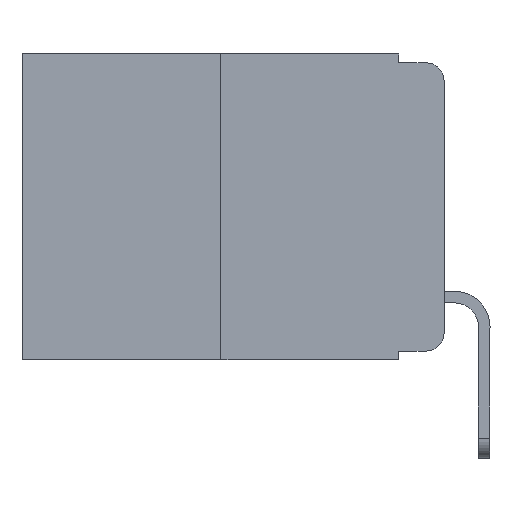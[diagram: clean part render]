
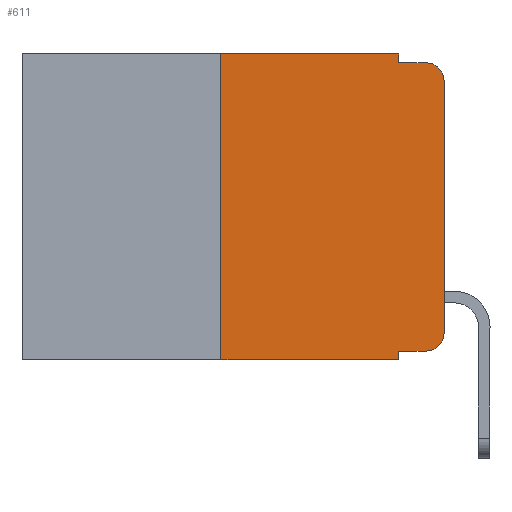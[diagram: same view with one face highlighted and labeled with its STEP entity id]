
A CAD part, left-side view. The second image highlights one B-rep face of the part: STEP entity #611.
In plain terms, the highlighted planar face has unit normal (-1, 0, 0).
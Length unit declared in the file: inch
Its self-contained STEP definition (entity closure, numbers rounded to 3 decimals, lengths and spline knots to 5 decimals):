
#88 = VECTOR ( 'NONE', #9686, 39.37008 ) ;
#611 = ADVANCED_FACE ( 'NONE', ( #10473 ), #3300, .F. ) ;
#733 = LINE ( 'NONE', #9210, #88 ) ;
#1097 = DIRECTION ( 'NONE',  ( 0., 0., 1. ) ) ;
#1259 = DIRECTION ( 'NONE',  ( -1., 0., 0. ) ) ;
#1465 = CARTESIAN_POINT ( 'NONE',  ( 0., 0.473, -0.343 ) ) ;
#1466 = EDGE_CURVE ( 'NONE', #6577, #6787, #733, .T. ) ;
#1718 = ORIENTED_EDGE ( 'NONE', *, *, #11756, .T. ) ;
#3211 = CARTESIAN_POINT ( 'NONE',  ( 0., 0.473, 0. ) ) ;
#3230 = VERTEX_POINT ( 'NONE', #4452 ) ;
#3300 = PLANE ( 'NONE',  #22395 ) ;
#3585 = ORIENTED_EDGE ( 'NONE', *, *, #6081, .T. ) ;
#3670 = LINE ( 'NONE', #19578, #22132 ) ;
#4152 = CARTESIAN_POINT ( 'NONE',  ( 0., 0.051, 0. ) ) ;
#4452 = CARTESIAN_POINT ( 'NONE',  ( 0., 0.051, -0.01 ) ) ;
#5296 = VERTEX_POINT ( 'NONE', #10024 ) ;
#5356 = CARTESIAN_POINT ( 'NONE',  ( 0., 0.02, -0.333 ) ) ;
#5412 = EDGE_CURVE ( 'NONE', #6280, #3230, #3670, .T. ) ;
#6081 = EDGE_CURVE ( 'NONE', #6577, #10014, #23718, .T. ) ;
#6172 = LINE ( 'NONE', #19785, #20274 ) ;
#6280 = VERTEX_POINT ( 'NONE', #22541 ) ;
#6577 = VERTEX_POINT ( 'NONE', #19228 ) ;
#6715 = EDGE_CURVE ( 'NONE', #3230, #21438, #17166, .T. ) ;
#6787 = VERTEX_POINT ( 'NONE', #16403 ) ;
#6849 = CARTESIAN_POINT ( 'NONE',  ( 0., 0.051, -0.01 ) ) ;
#6919 = ORIENTED_EDGE ( 'NONE', *, *, #9229, .T. ) ;
#6920 = DIRECTION ( 'NONE',  ( -1., 0., 0. ) ) ;
#7929 = LINE ( 'NONE', #4152, #16643 ) ;
#8415 = VECTOR ( 'NONE', #13838, 39.37008 ) ;
#9210 = CARTESIAN_POINT ( 'NONE',  ( 0., 0.25, 0. ) ) ;
#9229 = EDGE_CURVE ( 'NONE', #5296, #21438, #17628, .T. ) ;
#9271 = ORIENTED_EDGE ( 'NONE', *, *, #23041, .F. ) ;
#9686 = DIRECTION ( 'NONE',  ( 0., 0., 1. ) ) ;
#9834 = CARTESIAN_POINT ( 'NONE',  ( 0., 0.02, -0.01 ) ) ;
#9861 = ORIENTED_EDGE ( 'NONE', *, *, #18319, .T. ) ;
#10014 = VERTEX_POINT ( 'NONE', #17397 ) ;
#10024 = CARTESIAN_POINT ( 'NONE',  ( 0., 0., -0.03 ) ) ;
#10473 = FACE_OUTER_BOUND ( 'NONE', #21696, .T. ) ;
#11504 = DIRECTION ( 'NONE',  ( 0., -1., 0. ) ) ;
#11756 = EDGE_CURVE ( 'NONE', #23983, #5296, #6172, .T. ) ;
#11792 = DIRECTION ( 'NONE',  ( 0., 0., -1. ) ) ;
#11904 = ORIENTED_EDGE ( 'NONE', *, *, #6715, .F. ) ;
#12488 = ORIENTED_EDGE ( 'NONE', *, *, #5412, .F. ) ;
#12557 = CARTESIAN_POINT ( 'NONE',  ( 0., 0., -0.313 ) ) ;
#12733 = CARTESIAN_POINT ( 'NONE',  ( 0., 0.02, -0.03 ) ) ;
#13445 = CIRCLE ( 'NONE', #21872, 0.02 ) ;
#13838 = DIRECTION ( 'NONE',  ( 0., -1., 0. ) ) ;
#14300 = VECTOR ( 'NONE', #23679, 39.37008 ) ;
#14572 = LINE ( 'NONE', #15698, #8415 ) ;
#14627 = DIRECTION ( 'NONE',  ( 0., 0., -1. ) ) ;
#14845 = ORIENTED_EDGE ( 'NONE', *, *, #15960, .T. ) ;
#15241 = DIRECTION ( 'NONE',  ( 0., 0., -1. ) ) ;
#15698 = CARTESIAN_POINT ( 'NONE',  ( 0., 0.473, 0. ) ) ;
#15960 = EDGE_CURVE ( 'NONE', #22687, #23983, #13445, .T. ) ;
#16187 = DIRECTION ( 'NONE',  ( 1., 0., 0. ) ) ;
#16403 = CARTESIAN_POINT ( 'NONE',  ( 0., 0.25, 0. ) ) ;
#16643 = VECTOR ( 'NONE', #11792, 39.37008 ) ;
#16652 = VERTEX_POINT ( 'NONE', #23336 ) ;
#17031 = EDGE_CURVE ( 'NONE', #6787, #6280, #14572, .T. ) ;
#17166 = LINE ( 'NONE', #6849, #22403 ) ;
#17361 = ORIENTED_EDGE ( 'NONE', *, *, #17031, .F. ) ;
#17397 = CARTESIAN_POINT ( 'NONE',  ( 0., 0.051, -0.343 ) ) ;
#17628 = CIRCLE ( 'NONE', #20073, 0.02 ) ;
#17997 = CARTESIAN_POINT ( 'NONE',  ( 0., 0.02, -0.313 ) ) ;
#18319 = EDGE_CURVE ( 'NONE', #16652, #22687, #23109, .T. ) ;
#19228 = CARTESIAN_POINT ( 'NONE',  ( 0., 0.25, -0.343 ) ) ;
#19578 = CARTESIAN_POINT ( 'NONE',  ( 0., 0.051, 0. ) ) ;
#19717 = DIRECTION ( 'NONE',  ( 0., -1., 0. ) ) ;
#19773 = DIRECTION ( 'NONE',  ( 0., 0., -1. ) ) ;
#19785 = CARTESIAN_POINT ( 'NONE',  ( 0., 0., 0. ) ) ;
#20073 = AXIS2_PLACEMENT_3D ( 'NONE', #12733, #1259, #14627 ) ;
#20274 = VECTOR ( 'NONE', #1097, 39.37008 ) ;
#21384 = DIRECTION ( 'NONE',  ( 0., 0., -1. ) ) ;
#21438 = VERTEX_POINT ( 'NONE', #9834 ) ;
#21696 = EDGE_LOOP ( 'NONE', ( #1718, #6919, #11904, #12488, #17361, #22600, #3585, #9271, #9861, #14845 ) ) ;
#21872 = AXIS2_PLACEMENT_3D ( 'NONE', #17997, #6920, #19773 ) ;
#22020 = VECTOR ( 'NONE', #11504, 39.37008 ) ;
#22132 = VECTOR ( 'NONE', #21384, 39.37008 ) ;
#22284 = CARTESIAN_POINT ( 'NONE',  ( 0., 0.051, -0.333 ) ) ;
#22395 = AXIS2_PLACEMENT_3D ( 'NONE', #3211, #16187, #15241 ) ;
#22403 = VECTOR ( 'NONE', #19717, 39.37008 ) ;
#22541 = CARTESIAN_POINT ( 'NONE',  ( 0., 0.051, 0. ) ) ;
#22600 = ORIENTED_EDGE ( 'NONE', *, *, #1466, .F. ) ;
#22687 = VERTEX_POINT ( 'NONE', #5356 ) ;
#23041 = EDGE_CURVE ( 'NONE', #16652, #10014, #7929, .T. ) ;
#23109 = LINE ( 'NONE', #22284, #22020 ) ;
#23336 = CARTESIAN_POINT ( 'NONE',  ( 0., 0.051, -0.333 ) ) ;
#23679 = DIRECTION ( 'NONE',  ( 0., -1., 0. ) ) ;
#23718 = LINE ( 'NONE', #1465, #14300 ) ;
#23983 = VERTEX_POINT ( 'NONE', #12557 ) ;
